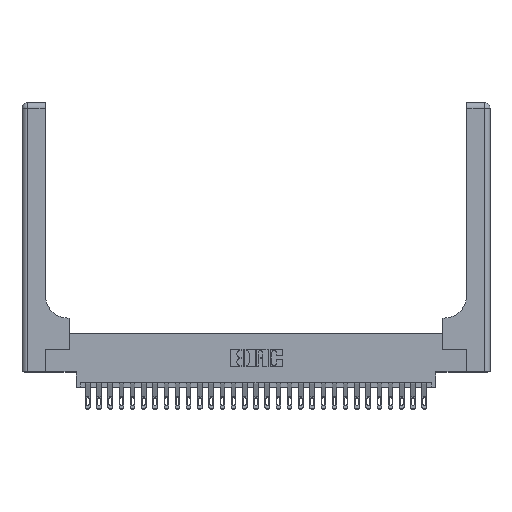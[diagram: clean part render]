
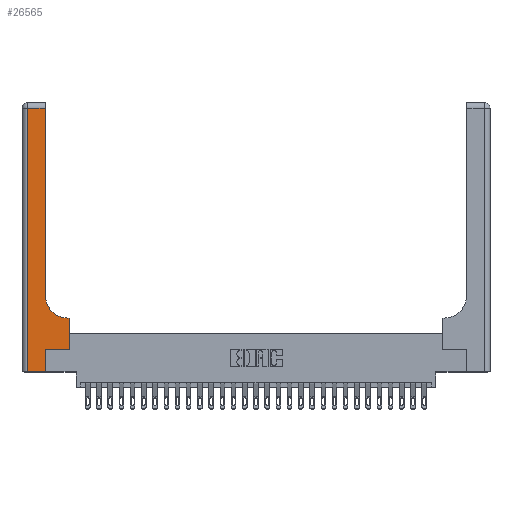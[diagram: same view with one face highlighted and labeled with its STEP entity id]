
A CAD part, top view. The second image highlights one B-rep face of the part: STEP entity #26565.
In plain terms, the highlighted planar face has unit normal (0, 0, 1).
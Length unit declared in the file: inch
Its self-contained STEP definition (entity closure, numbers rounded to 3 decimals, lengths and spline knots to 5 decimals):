
#311 = VERTEX_POINT ( 'NONE', #787 ) ;
#376 = LINE ( 'NONE', #24038, #25810 ) ;
#787 = CARTESIAN_POINT ( 'NONE',  ( 0.06, 0., 0.37 ) ) ;
#987 = EDGE_CURVE ( 'NONE', #12257, #6420, #8091, .T. ) ;
#1214 = EDGE_CURVE ( 'NONE', #6420, #8085, #12120, .T. ) ;
#1728 = LINE ( 'NONE', #1991, #14566 ) ;
#1991 = CARTESIAN_POINT ( 'NONE',  ( 0.528, 0.25, 0.37 ) ) ;
#2117 = CARTESIAN_POINT ( 'NONE',  ( 0.26, 2.94, 0.37 ) ) ;
#2906 = VECTOR ( 'NONE', #11013, 39.37008 ) ;
#2982 = LINE ( 'NONE', #6654, #2906 ) ;
#3405 = VERTEX_POINT ( 'NONE', #4850 ) ;
#4800 = CARTESIAN_POINT ( 'NONE',  ( 0.528, 0.25, 0.37 ) ) ;
#4850 = CARTESIAN_POINT ( 'NONE',  ( 0.06, 2.94, 0.37 ) ) ;
#4941 = VERTEX_POINT ( 'NONE', #2117 ) ;
#5360 = CARTESIAN_POINT ( 'NONE',  ( 0.265, 0.25, 0.37 ) ) ;
#5468 = LINE ( 'NONE', #14873, #23496 ) ;
#5827 = DIRECTION ( 'NONE',  ( -1., 0., 0. ) ) ;
#5955 = DIRECTION ( 'NONE',  ( 0., 0., -1. ) ) ;
#6362 = ORIENTED_EDGE ( 'NONE', *, *, #17991, .T. ) ;
#6382 = DIRECTION ( 'NONE',  ( 0., 1., 0. ) ) ;
#6420 = VERTEX_POINT ( 'NONE', #9056 ) ;
#6584 = LINE ( 'NONE', #27694, #21299 ) ;
#6649 = VERTEX_POINT ( 'NONE', #21365 ) ;
#6654 = CARTESIAN_POINT ( 'NONE',  ( 0.26, 3., 0.37 ) ) ;
#6930 = AXIS2_PLACEMENT_3D ( 'NONE', #27762, #5955, #14551 ) ;
#7495 = CARTESIAN_POINT ( 'NONE',  ( 0., 2.94, 0.37 ) ) ;
#7712 = EDGE_CURVE ( 'NONE', #4941, #3405, #27041, .T. ) ;
#8085 = VERTEX_POINT ( 'NONE', #4800 ) ;
#8091 = LINE ( 'NONE', #16682, #11167 ) ;
#8204 = CARTESIAN_POINT ( 'NONE',  ( 0., 3., 0.37 ) ) ;
#8764 = EDGE_LOOP ( 'NONE', ( #9116, #23915, #25716, #9553, #16756, #8916, #25122, #21622, #6362 ) ) ;
#8916 = ORIENTED_EDGE ( 'NONE', *, *, #1214, .T. ) ;
#9056 = CARTESIAN_POINT ( 'NONE',  ( 0.265, 0.25, 0.37 ) ) ;
#9116 = ORIENTED_EDGE ( 'NONE', *, *, #18157, .T. ) ;
#9553 = ORIENTED_EDGE ( 'NONE', *, *, #15387, .T. ) ;
#11013 = DIRECTION ( 'NONE',  ( 0., 1., 0. ) ) ;
#11167 = VECTOR ( 'NONE', #6382, 39.37008 ) ;
#11878 = CARTESIAN_POINT ( 'NONE',  ( 0.26, 0.85, 0.37 ) ) ;
#12120 = LINE ( 'NONE', #5360, #21533 ) ;
#12257 = VERTEX_POINT ( 'NONE', #26365 ) ;
#13348 = DIRECTION ( 'NONE',  ( 1., 0., 0. ) ) ;
#14445 = EDGE_CURVE ( 'NONE', #8085, #21527, #1728, .T. ) ;
#14475 = CARTESIAN_POINT ( 'NONE',  ( 0.528, 0.6, 0.37 ) ) ;
#14551 = DIRECTION ( 'NONE',  ( 1., 0., 0. ) ) ;
#14566 = VECTOR ( 'NONE', #18770, 39.37008 ) ;
#14703 = DIRECTION ( 'NONE',  ( 0., 0., -1. ) ) ;
#14873 = CARTESIAN_POINT ( 'NONE',  ( 0.06, 3., 0.37 ) ) ;
#15180 = VECTOR ( 'NONE', #24822, 39.37008 ) ;
#15387 = EDGE_CURVE ( 'NONE', #311, #12257, #376, .T. ) ;
#15898 = CIRCLE ( 'NONE', #6930, 0.25 ) ;
#16682 = CARTESIAN_POINT ( 'NONE',  ( 0.265, 0., 0.37 ) ) ;
#16756 = ORIENTED_EDGE ( 'NONE', *, *, #987, .T. ) ;
#17578 = DIRECTION ( 'NONE',  ( -1., 0., 0. ) ) ;
#17962 = FACE_OUTER_BOUND ( 'NONE', #8764, .T. ) ;
#17991 = EDGE_CURVE ( 'NONE', #6649, #25177, #15898, .T. ) ;
#18034 = DIRECTION ( 'NONE',  ( 1., 0., 0. ) ) ;
#18157 = EDGE_CURVE ( 'NONE', #25177, #4941, #2982, .T. ) ;
#18770 = DIRECTION ( 'NONE',  ( 0., 1., 0. ) ) ;
#21299 = VECTOR ( 'NONE', #17578, 39.37008 ) ;
#21365 = CARTESIAN_POINT ( 'NONE',  ( 0.51, 0.6, 0.37 ) ) ;
#21527 = VERTEX_POINT ( 'NONE', #14475 ) ;
#21533 = VECTOR ( 'NONE', #18034, 39.37008 ) ;
#21622 = ORIENTED_EDGE ( 'NONE', *, *, #27630, .T. ) ;
#23437 = DIRECTION ( 'NONE',  ( 0., -1., 0. ) ) ;
#23496 = VECTOR ( 'NONE', #23437, 39.37008 ) ;
#23517 = AXIS2_PLACEMENT_3D ( 'NONE', #8204, #14703, #5827 ) ;
#23915 = ORIENTED_EDGE ( 'NONE', *, *, #7712, .T. ) ;
#24038 = CARTESIAN_POINT ( 'NONE',  ( 0., 0., 0.37 ) ) ;
#24822 = DIRECTION ( 'NONE',  ( -1., 0., 0. ) ) ;
#25122 = ORIENTED_EDGE ( 'NONE', *, *, #14445, .T. ) ;
#25177 = VERTEX_POINT ( 'NONE', #11878 ) ;
#25716 = ORIENTED_EDGE ( 'NONE', *, *, #26221, .T. ) ;
#25810 = VECTOR ( 'NONE', #13348, 39.37008 ) ;
#26221 = EDGE_CURVE ( 'NONE', #3405, #311, #5468, .T. ) ;
#26365 = CARTESIAN_POINT ( 'NONE',  ( 0.265, 0., 0.37 ) ) ;
#26565 = ADVANCED_FACE ( 'NONE', ( #17962 ), #27470, .F. ) ;
#27041 = LINE ( 'NONE', #7495, #15180 ) ;
#27470 = PLANE ( 'NONE',  #23517 ) ;
#27630 = EDGE_CURVE ( 'NONE', #21527, #6649, #6584, .T. ) ;
#27694 = CARTESIAN_POINT ( 'NONE',  ( 0.26, 0.6, 0.37 ) ) ;
#27762 = CARTESIAN_POINT ( 'NONE',  ( 0.51, 0.85, 0.37 ) ) ;
